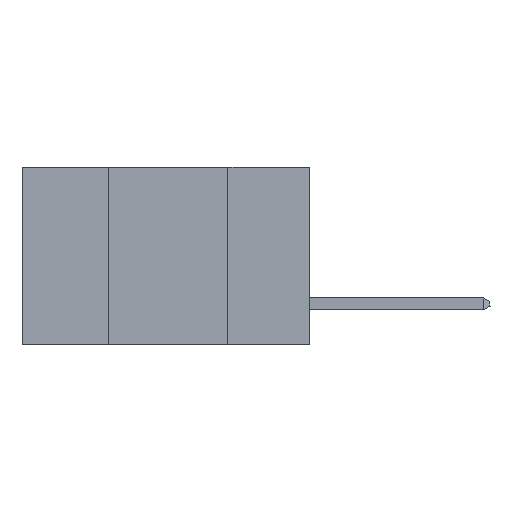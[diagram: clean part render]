
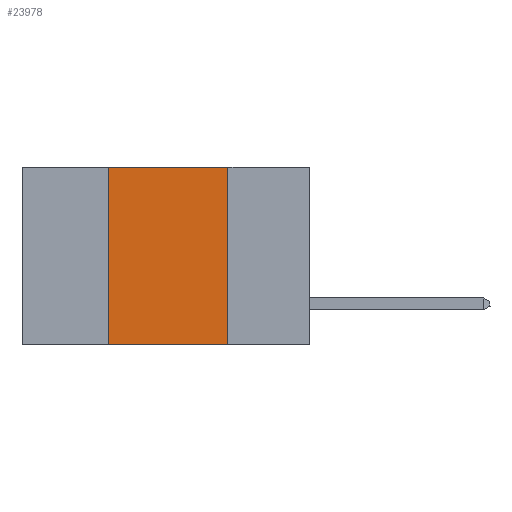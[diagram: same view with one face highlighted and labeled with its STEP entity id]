
A CAD part, left-side view. The second image highlights one B-rep face of the part: STEP entity #23978.
In plain terms, the highlighted planar face has unit normal (-1, 0, 0).
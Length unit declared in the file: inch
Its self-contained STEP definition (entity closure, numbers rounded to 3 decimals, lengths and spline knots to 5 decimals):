
#496 = CARTESIAN_POINT ( 'NONE',  ( 0., 0.6, 0. ) ) ;
#1171 = FACE_OUTER_BOUND ( 'NONE', #23078, .T. ) ;
#1429 = VECTOR ( 'NONE', #10278, 39.37008 ) ;
#1704 = CARTESIAN_POINT ( 'NONE',  ( 0., 0.17, 0. ) ) ;
#1890 = VECTOR ( 'NONE', #21047, 39.37008 ) ;
#2629 = EDGE_CURVE ( 'NONE', #12293, #24487, #18295, .T. ) ;
#2842 = EDGE_CURVE ( 'NONE', #15603, #7181, #26171, .T. ) ;
#3619 = LINE ( 'NONE', #496, #1429 ) ;
#3718 = DIRECTION ( 'NONE',  ( 0., 0., -1. ) ) ;
#4393 = CARTESIAN_POINT ( 'NONE',  ( 0., 0.42, -0.37 ) ) ;
#5427 = CARTESIAN_POINT ( 'NONE',  ( 0., 0.6, 0. ) ) ;
#7181 = VERTEX_POINT ( 'NONE', #18313 ) ;
#8549 = VECTOR ( 'NONE', #14624, 39.37008 ) ;
#10278 = DIRECTION ( 'NONE',  ( 0., -1., 0. ) ) ;
#11218 = CARTESIAN_POINT ( 'NONE',  ( 0., 0.17, 0. ) ) ;
#11562 = EDGE_CURVE ( 'NONE', #12293, #7181, #23371, .T. ) ;
#12233 = ORIENTED_EDGE ( 'NONE', *, *, #2629, .F. ) ;
#12293 = VERTEX_POINT ( 'NONE', #4393 ) ;
#12336 = ORIENTED_EDGE ( 'NONE', *, *, #15341, .F. ) ;
#12590 = VECTOR ( 'NONE', #3718, 39.37008 ) ;
#13565 = DIRECTION ( 'NONE',  ( 1., 0., 0. ) ) ;
#14624 = DIRECTION ( 'NONE',  ( 0., -1., 0. ) ) ;
#15341 = EDGE_CURVE ( 'NONE', #24487, #15603, #3619, .T. ) ;
#15603 = VERTEX_POINT ( 'NONE', #11218 ) ;
#15656 = DIRECTION ( 'NONE',  ( 0., 0., -1. ) ) ;
#15955 = CARTESIAN_POINT ( 'NONE',  ( 0., 0.42, 0. ) ) ;
#16705 = ORIENTED_EDGE ( 'NONE', *, *, #11562, .T. ) ;
#18295 = LINE ( 'NONE', #20884, #1890 ) ;
#18313 = CARTESIAN_POINT ( 'NONE',  ( 0., 0.17, -0.37 ) ) ;
#20636 = AXIS2_PLACEMENT_3D ( 'NONE', #5427, #13565, #15656 ) ;
#20884 = CARTESIAN_POINT ( 'NONE',  ( 0., 0.42, 0. ) ) ;
#21047 = DIRECTION ( 'NONE',  ( 0., 0., 1. ) ) ;
#22804 = CARTESIAN_POINT ( 'NONE',  ( 0., 0.6, -0.37 ) ) ;
#23078 = EDGE_LOOP ( 'NONE', ( #24481, #12336, #12233, #16705 ) ) ;
#23371 = LINE ( 'NONE', #22804, #8549 ) ;
#23598 = PLANE ( 'NONE',  #20636 ) ;
#23978 = ADVANCED_FACE ( 'NONE', ( #1171 ), #23598, .F. ) ;
#24481 = ORIENTED_EDGE ( 'NONE', *, *, #2842, .F. ) ;
#24487 = VERTEX_POINT ( 'NONE', #15955 ) ;
#26171 = LINE ( 'NONE', #1704, #12590 ) ;
